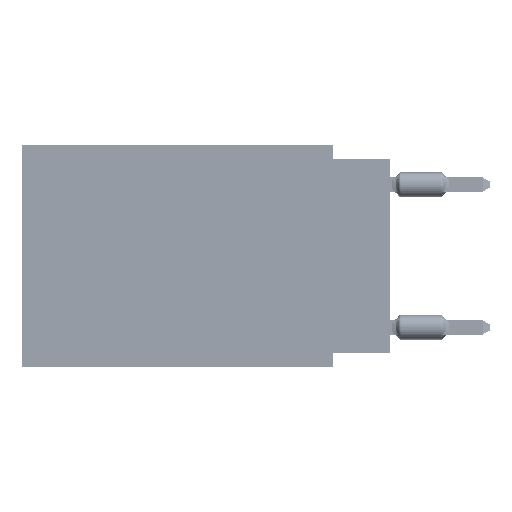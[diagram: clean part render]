
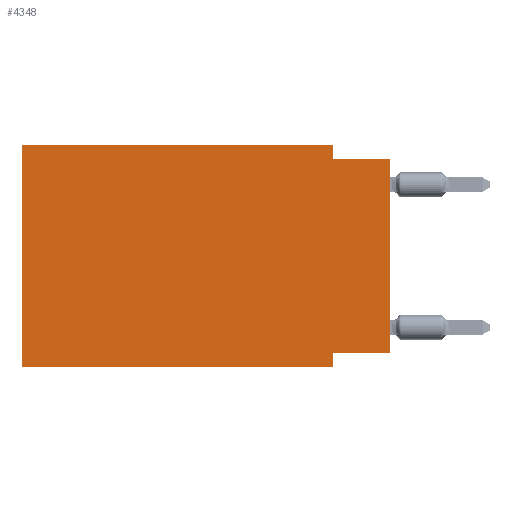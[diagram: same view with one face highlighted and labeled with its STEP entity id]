
A CAD part, left-side view. The second image highlights one B-rep face of the part: STEP entity #4348.
In plain terms, the highlighted planar face has unit normal (-1, 0, 0).
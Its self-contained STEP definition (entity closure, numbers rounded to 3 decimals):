
#2098 = EDGE_CURVE ( 'NONE', #3324, #71903, #33863, .T. ) ;
#2760 = DIRECTION ( 'NONE',  ( 1., 0., 0. ) ) ;
#3324 = VERTEX_POINT ( 'NONE', #22179 ) ;
#3767 = VECTOR ( 'NONE', #13405, 1000. ) ;
#3922 = EDGE_LOOP ( 'NONE', ( #6906, #29941, #51957, #71423, #49267, #62047, #59845, #61102 ) ) ;
#4167 = VECTOR ( 'NONE', #55369, 1000. ) ;
#4348 = ADVANCED_FACE ( 'NONE', ( #36786 ), #31895, .F. ) ;
#6906 = ORIENTED_EDGE ( 'NONE', *, *, #2098, .T. ) ;
#7226 = VECTOR ( 'NONE', #7867, 1000. ) ;
#7867 = DIRECTION ( 'NONE',  ( 0., 0., -1. ) ) ;
#8475 = CARTESIAN_POINT ( 'NONE',  ( 0., 16.383, 0. ) ) ;
#10051 = CARTESIAN_POINT ( 'NONE',  ( 0., 0., 0. ) ) ;
#11625 = AXIS2_PLACEMENT_3D ( 'NONE', #13758, #2760, #14886 ) ;
#11649 = VECTOR ( 'NONE', #66913, 1000. ) ;
#13251 = VERTEX_POINT ( 'NONE', #55880 ) ;
#13405 = DIRECTION ( 'NONE',  ( 0., -1., 0. ) ) ;
#13758 = CARTESIAN_POINT ( 'NONE',  ( 0., 16.383, 0. ) ) ;
#14886 = DIRECTION ( 'NONE',  ( 0., 0., -1. ) ) ;
#15471 = VERTEX_POINT ( 'NONE', #27427 ) ;
#17234 = CARTESIAN_POINT ( 'NONE',  ( 0., 0., -0.635 ) ) ;
#18817 = EDGE_CURVE ( 'NONE', #36181, #36067, #22226, .T. ) ;
#19778 = CARTESIAN_POINT ( 'NONE',  ( 0., 16.383, 0. ) ) ;
#19779 = DIRECTION ( 'NONE',  ( 0., -1., 0. ) ) ;
#22179 = CARTESIAN_POINT ( 'NONE',  ( 0., 0., -9.271 ) ) ;
#22226 = LINE ( 'NONE', #33187, #51605 ) ;
#23668 = EDGE_CURVE ( 'NONE', #31107, #13251, #71282, .T. ) ;
#24252 = VECTOR ( 'NONE', #19779, 1000. ) ;
#24716 = EDGE_CURVE ( 'NONE', #15471, #71903, #60492, .T. ) ;
#27252 = EDGE_CURVE ( 'NONE', #36067, #15471, #73335, .T. ) ;
#27427 = CARTESIAN_POINT ( 'NONE',  ( 0., 2.54, -0.635 ) ) ;
#29855 = VECTOR ( 'NONE', #48432, 1000. ) ;
#29941 = ORIENTED_EDGE ( 'NONE', *, *, #24716, .F. ) ;
#31107 = VERTEX_POINT ( 'NONE', #67076 ) ;
#31895 = PLANE ( 'NONE',  #11625 ) ;
#31918 = CARTESIAN_POINT ( 'NONE',  ( 0., 2.54, 0. ) ) ;
#33187 = CARTESIAN_POINT ( 'NONE',  ( 0., 16.383, 0. ) ) ;
#33863 = LINE ( 'NONE', #10051, #4167 ) ;
#36067 = VERTEX_POINT ( 'NONE', #31918 ) ;
#36181 = VERTEX_POINT ( 'NONE', #8475 ) ;
#36786 = FACE_OUTER_BOUND ( 'NONE', #3922, .T. ) ;
#38141 = VERTEX_POINT ( 'NONE', #73136 ) ;
#38230 = LINE ( 'NONE', #19778, #29855 ) ;
#40341 = EDGE_CURVE ( 'NONE', #38141, #36181, #38230, .T. ) ;
#42083 = LINE ( 'NONE', #43191, #3767 ) ;
#43191 = CARTESIAN_POINT ( 'NONE',  ( 0., 16.383, -9.906 ) ) ;
#43350 = CARTESIAN_POINT ( 'NONE',  ( 0., 2.54, -9.906 ) ) ;
#45965 = DIRECTION ( 'NONE',  ( 0., 1., 0. ) ) ;
#48432 = DIRECTION ( 'NONE',  ( 0., 0., 1. ) ) ;
#49267 = ORIENTED_EDGE ( 'NONE', *, *, #40341, .F. ) ;
#51605 = VECTOR ( 'NONE', #56160, 1000. ) ;
#51957 = ORIENTED_EDGE ( 'NONE', *, *, #27252, .F. ) ;
#55369 = DIRECTION ( 'NONE',  ( 0., 0., 1. ) ) ;
#55880 = CARTESIAN_POINT ( 'NONE',  ( 0., 2.54, -9.906 ) ) ;
#56160 = DIRECTION ( 'NONE',  ( 0., -1., 0. ) ) ;
#59845 = ORIENTED_EDGE ( 'NONE', *, *, #23668, .F. ) ;
#60492 = LINE ( 'NONE', #71437, #24252 ) ;
#61102 = ORIENTED_EDGE ( 'NONE', *, *, #68263, .F. ) ;
#62047 = ORIENTED_EDGE ( 'NONE', *, *, #70784, .T. ) ;
#66913 = DIRECTION ( 'NONE',  ( 0., 0., -1. ) ) ;
#67076 = CARTESIAN_POINT ( 'NONE',  ( 0., 2.54, -9.271 ) ) ;
#68263 = EDGE_CURVE ( 'NONE', #3324, #31107, #73549, .T. ) ;
#68613 = CARTESIAN_POINT ( 'NONE',  ( 0., 0., -9.271 ) ) ;
#70784 = EDGE_CURVE ( 'NONE', #38141, #13251, #42083, .T. ) ;
#71282 = LINE ( 'NONE', #43350, #7226 ) ;
#71423 = ORIENTED_EDGE ( 'NONE', *, *, #18817, .F. ) ;
#71437 = CARTESIAN_POINT ( 'NONE',  ( 0., 0., -0.635 ) ) ;
#71903 = VERTEX_POINT ( 'NONE', #17234 ) ;
#72112 = VECTOR ( 'NONE', #45965, 1000. ) ;
#73136 = CARTESIAN_POINT ( 'NONE',  ( 0., 16.383, -9.906 ) ) ;
#73335 = LINE ( 'NONE', #73699, #11649 ) ;
#73549 = LINE ( 'NONE', #68613, #72112 ) ;
#73699 = CARTESIAN_POINT ( 'NONE',  ( 0., 2.54, 0. ) ) ;
